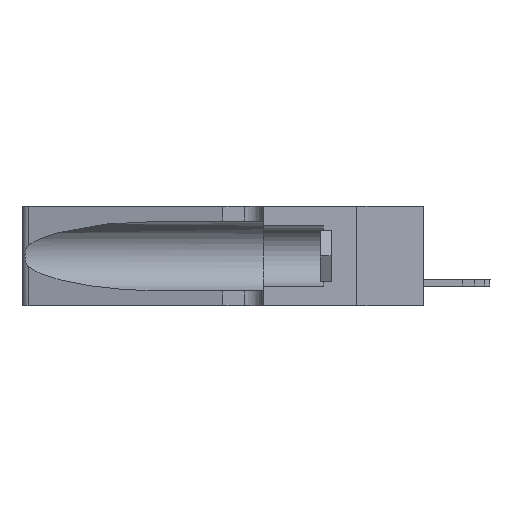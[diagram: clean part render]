
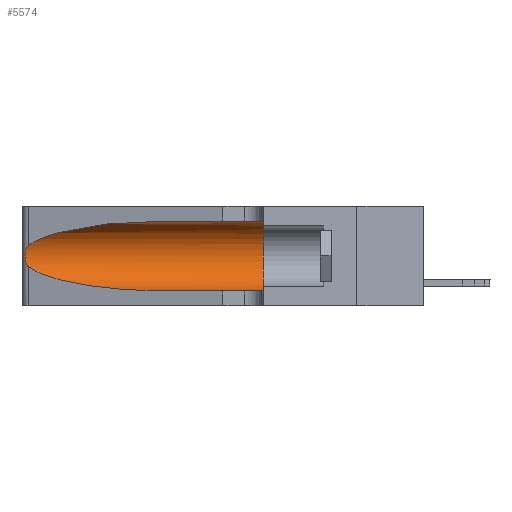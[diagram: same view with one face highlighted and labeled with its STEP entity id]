
A CAD part, left-side view. The second image highlights one B-rep face of the part: STEP entity #5574.
In plain terms, the highlighted cylindrical face has radius 3.308 mm (diameter 6.617 mm), a partial arc.
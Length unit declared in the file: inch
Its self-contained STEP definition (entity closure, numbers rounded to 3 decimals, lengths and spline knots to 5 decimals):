
#800 =( BOUNDED_CURVE ( )  B_SPLINE_CURVE ( 3, ( #15893, #8822, #8883, #8936 ),
 .UNSPECIFIED., .F., .F. ) 
 B_SPLINE_CURVE_WITH_KNOTS ( ( 4, 4 ),
 ( 3.44316, 4.71239 ),
 .UNSPECIFIED. ) 
 CURVE ( )  GEOMETRIC_REPRESENTATION_ITEM ( )  RATIONAL_B_SPLINE_CURVE ( ( 1., 0.87, 0.87, 1. ) ) 
 REPRESENTATION_ITEM ( '' )  );
#933 = VECTOR ( 'NONE', #11518, 39.37008 ) ;
#1424 = CARTESIAN_POINT ( 'NONE',  ( 0.25555, 1.22994, 0.2215 ) ) ;
#1779 = DIRECTION ( 'NONE',  ( 0., -1., 0. ) ) ;
#1936 = DIRECTION ( 'NONE',  ( 0., 0., 1. ) ) ;
#2095 = VERTEX_POINT ( 'NONE', #11229 ) ;
#2285 = VECTOR ( 'NONE', #1779, 39.37008 ) ;
#2613 = CARTESIAN_POINT ( 'NONE',  ( 0.26017, 1.23833, 0.17102 ) ) ;
#2866 = CARTESIAN_POINT ( 'NONE',  ( 0.25555, 1.22993, 0.14849 ) ) ;
#2869 = CARTESIAN_POINT ( 'NONE',  ( 0.1305, 1.61858, 0.05475 ) ) ;
#3308 = CIRCLE ( 'NONE', #6848, 0.13025 ) ;
#3756 = ORIENTED_EDGE ( 'NONE', *, *, #9657, .F. ) ;
#4086 = CARTESIAN_POINT ( 'NONE',  ( 0.25639, 1.23186, 0.15144 ) ) ;
#4142 = CARTESIAN_POINT ( 'NONE',  ( 0.25789, 1.23486, 0.15765 ) ) ;
#4166 = CARTESIAN_POINT ( 'NONE',  ( 0.1305, 0.72297, 0.31525 ) ) ;
#4202 = FACE_OUTER_BOUND ( 'NONE', #16645, .T. ) ;
#4210 = CARTESIAN_POINT ( 'NONE',  ( 0.25854, 1.2359, 0.20912 ) ) ;
#4288 = AXIS2_PLACEMENT_3D ( 'NONE', #16006, #11537, #15809 ) ;
#4323 = VERTEX_POINT ( 'NONE', #15102 ) ;
#4738 = B_SPLINE_CURVE_WITH_KNOTS ( 'NONE', 3,
 ( #18842, #1424, #8423, #7088, #4210, #11586, #17328, #9920, #2613, #5498, #4142, #4086, #2866, #17270 ),
 .UNSPECIFIED., .F., .F.,
 ( 4, 2, 2, 2, 2, 2, 4 ),
 ( 0., 0.00027, 0.00053, 0.00107, 0.0016, 0.00187, 0.00214 ),
 .UNSPECIFIED. ) ;
#4993 = VERTEX_POINT ( 'NONE', #12364 ) ;
#5498 = CARTESIAN_POINT ( 'NONE',  ( 0.25856, 1.23593, 0.16098 ) ) ;
#5574 = ADVANCED_FACE ( 'NONE', ( #4202 ), #17172, .F. ) ;
#6322 = CARTESIAN_POINT ( 'NONE',  ( 0.1305, 0.35, 0.185 ) ) ;
#6848 = AXIS2_PLACEMENT_3D ( 'NONE', #6322, #10451, #1936 ) ;
#7088 = CARTESIAN_POINT ( 'NONE',  ( 0.25787, 1.23484, 0.2124 ) ) ;
#8423 = CARTESIAN_POINT ( 'NONE',  ( 0.25639, 1.23184, 0.21858 ) ) ;
#8822 = CARTESIAN_POINT ( 'NONE',  ( 0.2373, 1.15595, 0.08982 ) ) ;
#8883 = CARTESIAN_POINT ( 'NONE',  ( 0.18966, 0.96281, 0.05475 ) ) ;
#8936 = CARTESIAN_POINT ( 'NONE',  ( 0.1305, 0.72297, 0.05475 ) ) ;
#9657 = EDGE_CURVE ( 'NONE', #10469, #4993, #17977, .T. ) ;
#9735 = CARTESIAN_POINT ( 'NONE',  ( 0.25487, 1.22718, 0.22369 ) ) ;
#9790 = EDGE_CURVE ( 'NONE', #10469, #2095, #16761, .T. ) ;
#9920 = CARTESIAN_POINT ( 'NONE',  ( 0.26075, 1.23896, 0.178 ) ) ;
#10203 = ORIENTED_EDGE ( 'NONE', *, *, #18354, .T. ) ;
#10451 = DIRECTION ( 'NONE',  ( 0., 1., 0. ) ) ;
#10469 = VERTEX_POINT ( 'NONE', #4166 ) ;
#10780 = CARTESIAN_POINT ( 'NONE',  ( 0.25487, 1.22718, 0.14631 ) ) ;
#11229 = CARTESIAN_POINT ( 'NONE',  ( 0.25487, 1.22718, 0.22369 ) ) ;
#11518 = DIRECTION ( 'NONE',  ( 0., -1., 0. ) ) ;
#11537 = DIRECTION ( 'NONE',  ( 0., -1., 0. ) ) ;
#11586 = CARTESIAN_POINT ( 'NONE',  ( 0.26018, 1.23835, 0.19895 ) ) ;
#12364 = CARTESIAN_POINT ( 'NONE',  ( 0.1305, 0.35, 0.31525 ) ) ;
#12927 = EDGE_CURVE ( 'NONE', #2095, #16719, #4738, .T. ) ;
#13794 = CARTESIAN_POINT ( 'NONE',  ( 0.18966, 0.96281, 0.31525 ) ) ;
#13873 = VERTEX_POINT ( 'NONE', #13952 ) ;
#13952 = CARTESIAN_POINT ( 'NONE',  ( 0.1305, 0.72297, 0.05475 ) ) ;
#14748 = EDGE_CURVE ( 'NONE', #13873, #4323, #15952, .T. ) ;
#15102 = CARTESIAN_POINT ( 'NONE',  ( 0.1305, 0.35, 0.05475 ) ) ;
#15397 = CARTESIAN_POINT ( 'NONE',  ( 0.2373, 1.15595, 0.28018 ) ) ;
#15809 = DIRECTION ( 'NONE',  ( 0., 0., -1. ) ) ;
#15893 = CARTESIAN_POINT ( 'NONE',  ( 0.25487, 1.22718, 0.14631 ) ) ;
#15952 = LINE ( 'NONE', #2869, #933 ) ;
#15966 = ORIENTED_EDGE ( 'NONE', *, *, #17250, .F. ) ;
#16006 = CARTESIAN_POINT ( 'NONE',  ( 0.1305, 1.61858, 0.185 ) ) ;
#16431 = ORIENTED_EDGE ( 'NONE', *, *, #14748, .T. ) ;
#16645 = EDGE_LOOP ( 'NONE', ( #18862, #17927, #10203, #16431, #15966, #3756 ) ) ;
#16719 = VERTEX_POINT ( 'NONE', #10780 ) ;
#16761 =( BOUNDED_CURVE ( )  B_SPLINE_CURVE ( 3, ( #18018, #13794, #15397, #9735 ),
 .UNSPECIFIED., .F., .F. ) 
 B_SPLINE_CURVE_WITH_KNOTS ( ( 4, 4 ),
 ( 1.5708, 2.84003 ),
 .UNSPECIFIED. ) 
 CURVE ( )  GEOMETRIC_REPRESENTATION_ITEM ( )  RATIONAL_B_SPLINE_CURVE ( ( 1., 0.87, 0.87, 1. ) ) 
 REPRESENTATION_ITEM ( '' )  );
#17172 = CYLINDRICAL_SURFACE ( 'NONE', #4288, 0.13025 ) ;
#17250 = EDGE_CURVE ( 'NONE', #4993, #4323, #3308, .T. ) ;
#17270 = CARTESIAN_POINT ( 'NONE',  ( 0.25487, 1.22718, 0.14631 ) ) ;
#17328 = CARTESIAN_POINT ( 'NONE',  ( 0.26075, 1.23896, 0.19203 ) ) ;
#17677 = CARTESIAN_POINT ( 'NONE',  ( 0.1305, 1.61858, 0.31525 ) ) ;
#17927 = ORIENTED_EDGE ( 'NONE', *, *, #12927, .T. ) ;
#17977 = LINE ( 'NONE', #17677, #2285 ) ;
#18018 = CARTESIAN_POINT ( 'NONE',  ( 0.1305, 0.72297, 0.31525 ) ) ;
#18354 = EDGE_CURVE ( 'NONE', #16719, #13873, #800, .T. ) ;
#18842 = CARTESIAN_POINT ( 'NONE',  ( 0.25487, 1.22718, 0.22369 ) ) ;
#18862 = ORIENTED_EDGE ( 'NONE', *, *, #9790, .T. ) ;
